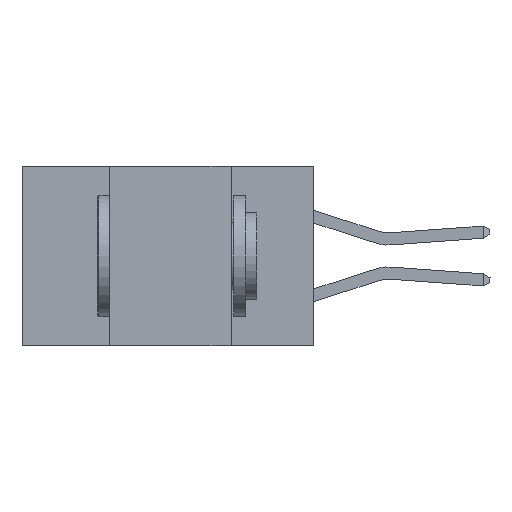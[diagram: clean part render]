
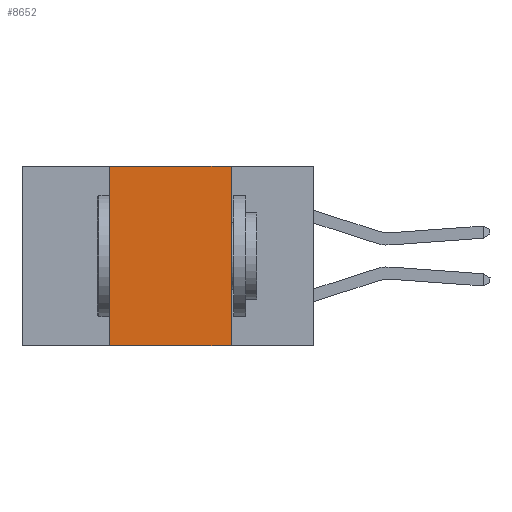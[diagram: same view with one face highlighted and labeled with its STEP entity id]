
A CAD part, left-side view. The second image highlights one B-rep face of the part: STEP entity #8652.
In plain terms, the highlighted planar face has unit normal (-1, 0, 0).
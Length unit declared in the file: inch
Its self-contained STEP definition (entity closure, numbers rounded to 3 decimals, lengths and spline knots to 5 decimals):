
#1202 = VECTOR ( 'NONE', #5465, 39.37008 ) ;
#1602 = DIRECTION ( 'NONE',  ( 0., 0., -1. ) ) ;
#2334 = VERTEX_POINT ( 'NONE', #13306 ) ;
#2621 = DIRECTION ( 'NONE',  ( 0., -1., 0. ) ) ;
#2627 = AXIS2_PLACEMENT_3D ( 'NONE', #13110, #14482, #6202 ) ;
#2690 = CARTESIAN_POINT ( 'NONE',  ( 0., 0.6, 0. ) ) ;
#3325 = PLANE ( 'NONE',  #2627 ) ;
#3583 = EDGE_CURVE ( 'NONE', #2334, #12516, #9710, .T. ) ;
#4719 = LINE ( 'NONE', #2690, #12596 ) ;
#5183 = EDGE_CURVE ( 'NONE', #12386, #16990, #4719, .T. ) ;
#5465 = DIRECTION ( 'NONE',  ( 0., 0., 1. ) ) ;
#6202 = DIRECTION ( 'NONE',  ( 0., 0., -1. ) ) ;
#6373 = FACE_OUTER_BOUND ( 'NONE', #12252, .T. ) ;
#6477 = EDGE_CURVE ( 'NONE', #2334, #12386, #12548, .T. ) ;
#8652 = ADVANCED_FACE ( 'NONE', ( #6373 ), #3325, .F. ) ;
#8795 = LINE ( 'NONE', #10187, #12479 ) ;
#9331 = CARTESIAN_POINT ( 'NONE',  ( 0., 0.42, 0. ) ) ;
#9710 = LINE ( 'NONE', #14479, #10152 ) ;
#10152 = VECTOR ( 'NONE', #14402, 39.37008 ) ;
#10187 = CARTESIAN_POINT ( 'NONE',  ( 0., 0.17, 0. ) ) ;
#11076 = CARTESIAN_POINT ( 'NONE',  ( 0., 0.17, 0. ) ) ;
#11337 = ORIENTED_EDGE ( 'NONE', *, *, #12069, .F. ) ;
#12069 = EDGE_CURVE ( 'NONE', #16990, #12516, #8795, .T. ) ;
#12252 = EDGE_LOOP ( 'NONE', ( #11337, #12387, #16020, #13357 ) ) ;
#12386 = VERTEX_POINT ( 'NONE', #9331 ) ;
#12387 = ORIENTED_EDGE ( 'NONE', *, *, #5183, .F. ) ;
#12409 = CARTESIAN_POINT ( 'NONE',  ( 0., 0.42, 0. ) ) ;
#12479 = VECTOR ( 'NONE', #1602, 39.37008 ) ;
#12516 = VERTEX_POINT ( 'NONE', #15053 ) ;
#12548 = LINE ( 'NONE', #12409, #1202 ) ;
#12596 = VECTOR ( 'NONE', #2621, 39.37008 ) ;
#13110 = CARTESIAN_POINT ( 'NONE',  ( 0., 0.6, 0. ) ) ;
#13306 = CARTESIAN_POINT ( 'NONE',  ( 0., 0.42, -0.37 ) ) ;
#13357 = ORIENTED_EDGE ( 'NONE', *, *, #3583, .T. ) ;
#14402 = DIRECTION ( 'NONE',  ( 0., -1., 0. ) ) ;
#14479 = CARTESIAN_POINT ( 'NONE',  ( 0., 0.6, -0.37 ) ) ;
#14482 = DIRECTION ( 'NONE',  ( 1., 0., 0. ) ) ;
#15053 = CARTESIAN_POINT ( 'NONE',  ( 0., 0.17, -0.37 ) ) ;
#16020 = ORIENTED_EDGE ( 'NONE', *, *, #6477, .F. ) ;
#16990 = VERTEX_POINT ( 'NONE', #11076 ) ;
